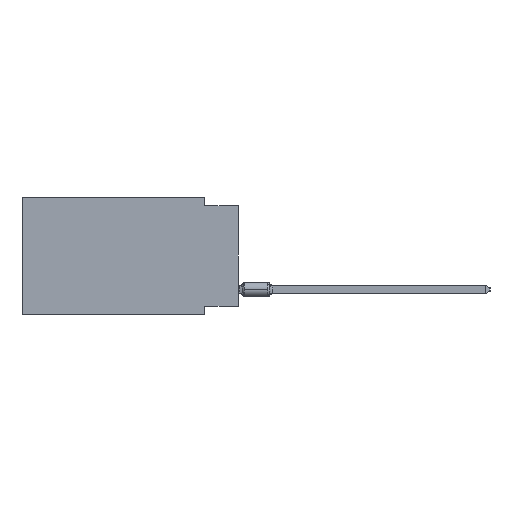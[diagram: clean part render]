
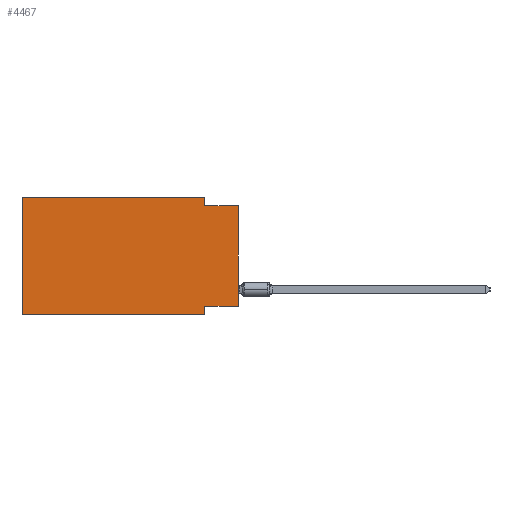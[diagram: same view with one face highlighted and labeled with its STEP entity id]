
A CAD part, left-side view. The second image highlights one B-rep face of the part: STEP entity #4467.
In plain terms, the highlighted planar face has unit normal (-1, 0, 0).
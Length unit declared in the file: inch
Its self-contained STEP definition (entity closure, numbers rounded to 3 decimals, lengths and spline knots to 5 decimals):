
#11 = EDGE_CURVE ( 'NONE', #9144, #3009, #10147, .T. ) ;
#257 = CARTESIAN_POINT ( 'NONE',  ( 0., 0.645, 0. ) ) ;
#441 = CARTESIAN_POINT ( 'NONE',  ( 0., 0.1, -0.35 ) ) ;
#1061 = CARTESIAN_POINT ( 'NONE',  ( 0., 0.645, 0. ) ) ;
#1455 = FACE_OUTER_BOUND ( 'NONE', #5519, .T. ) ;
#2719 = EDGE_CURVE ( 'NONE', #9144, #8437, #14019, .T. ) ;
#2904 = CARTESIAN_POINT ( 'NONE',  ( 0., 0.645, 0. ) ) ;
#3009 = VERTEX_POINT ( 'NONE', #11769 ) ;
#3691 = EDGE_CURVE ( 'NONE', #12762, #14898, #10956, .T. ) ;
#4150 = EDGE_CURVE ( 'NONE', #14898, #8437, #11173, .T. ) ;
#4467 = ADVANCED_FACE ( 'NONE', ( #1455 ), #18642, .F. ) ;
#4800 = DIRECTION ( 'NONE',  ( 0., 0., 1. ) ) ;
#4844 = ORIENTED_EDGE ( 'NONE', *, *, #5484, .F. ) ;
#5359 = CARTESIAN_POINT ( 'NONE',  ( 0., 0.1, -0.35 ) ) ;
#5396 = VECTOR ( 'NONE', #8864, 39.37008 ) ;
#5484 = EDGE_CURVE ( 'NONE', #23188, #22217, #22740, .T. ) ;
#5519 = EDGE_LOOP ( 'NONE', ( #13913, #9122, #12208, #10327, #4844, #9308, #16937, #17018 ) ) ;
#5646 = DIRECTION ( 'NONE',  ( 0., -1., 0. ) ) ;
#6126 = VECTOR ( 'NONE', #21265, 39.37008 ) ;
#6342 = VECTOR ( 'NONE', #19729, 39.37008 ) ;
#7537 = AXIS2_PLACEMENT_3D ( 'NONE', #16552, #18160, #20490 ) ;
#7762 = EDGE_CURVE ( 'NONE', #22217, #12762, #12457, .T. ) ;
#8126 = VECTOR ( 'NONE', #4800, 39.37008 ) ;
#8182 = CARTESIAN_POINT ( 'NONE',  ( 0., 0., -0.325 ) ) ;
#8437 = VERTEX_POINT ( 'NONE', #23218 ) ;
#8546 = EDGE_CURVE ( 'NONE', #3009, #16644, #9035, .T. ) ;
#8864 = DIRECTION ( 'NONE',  ( 0., -1., 0. ) ) ;
#9035 = LINE ( 'NONE', #5359, #9042 ) ;
#9042 = VECTOR ( 'NONE', #16178, 39.37008 ) ;
#9122 = ORIENTED_EDGE ( 'NONE', *, *, #4150, .F. ) ;
#9144 = VERTEX_POINT ( 'NONE', #13313 ) ;
#9308 = ORIENTED_EDGE ( 'NONE', *, *, #18975, .T. ) ;
#10147 = LINE ( 'NONE', #8182, #15173 ) ;
#10327 = ORIENTED_EDGE ( 'NONE', *, *, #7762, .F. ) ;
#10956 = LINE ( 'NONE', #12926, #20445 ) ;
#11173 = LINE ( 'NONE', #12654, #23988 ) ;
#11769 = CARTESIAN_POINT ( 'NONE',  ( 0., 0.1, -0.325 ) ) ;
#12208 = ORIENTED_EDGE ( 'NONE', *, *, #3691, .F. ) ;
#12442 = CARTESIAN_POINT ( 'NONE',  ( 0., 0.645, -0.35 ) ) ;
#12457 = LINE ( 'NONE', #2904, #6342 ) ;
#12654 = CARTESIAN_POINT ( 'NONE',  ( 0., 0., -0.025 ) ) ;
#12762 = VERTEX_POINT ( 'NONE', #21987 ) ;
#12926 = CARTESIAN_POINT ( 'NONE',  ( 0., 0.1, 0. ) ) ;
#13313 = CARTESIAN_POINT ( 'NONE',  ( 0., 0., -0.325 ) ) ;
#13913 = ORIENTED_EDGE ( 'NONE', *, *, #2719, .T. ) ;
#14019 = LINE ( 'NONE', #19914, #8126 ) ;
#14898 = VERTEX_POINT ( 'NONE', #23820 ) ;
#15173 = VECTOR ( 'NONE', #15794, 39.37008 ) ;
#15794 = DIRECTION ( 'NONE',  ( 0., 1., 0. ) ) ;
#16178 = DIRECTION ( 'NONE',  ( 0., 0., -1. ) ) ;
#16552 = CARTESIAN_POINT ( 'NONE',  ( 0., 0.645, 0. ) ) ;
#16644 = VERTEX_POINT ( 'NONE', #441 ) ;
#16937 = ORIENTED_EDGE ( 'NONE', *, *, #8546, .F. ) ;
#17018 = ORIENTED_EDGE ( 'NONE', *, *, #11, .F. ) ;
#18160 = DIRECTION ( 'NONE',  ( 1., 0., 0. ) ) ;
#18642 = PLANE ( 'NONE',  #7537 ) ;
#18975 = EDGE_CURVE ( 'NONE', #23188, #16644, #24131, .T. ) ;
#19729 = DIRECTION ( 'NONE',  ( 0., -1., 0. ) ) ;
#19914 = CARTESIAN_POINT ( 'NONE',  ( 0., 0., 0. ) ) ;
#20181 = DIRECTION ( 'NONE',  ( 0., 0., -1. ) ) ;
#20445 = VECTOR ( 'NONE', #20181, 39.37008 ) ;
#20490 = DIRECTION ( 'NONE',  ( 0., 0., -1. ) ) ;
#21265 = DIRECTION ( 'NONE',  ( 0., 0., 1. ) ) ;
#21987 = CARTESIAN_POINT ( 'NONE',  ( 0., 0.1, 0. ) ) ;
#22217 = VERTEX_POINT ( 'NONE', #1061 ) ;
#22740 = LINE ( 'NONE', #257, #6126 ) ;
#23078 = CARTESIAN_POINT ( 'NONE',  ( 0., 0.645, -0.35 ) ) ;
#23188 = VERTEX_POINT ( 'NONE', #23078 ) ;
#23218 = CARTESIAN_POINT ( 'NONE',  ( 0., 0., -0.025 ) ) ;
#23820 = CARTESIAN_POINT ( 'NONE',  ( 0., 0.1, -0.025 ) ) ;
#23988 = VECTOR ( 'NONE', #5646, 39.37008 ) ;
#24131 = LINE ( 'NONE', #12442, #5396 ) ;
